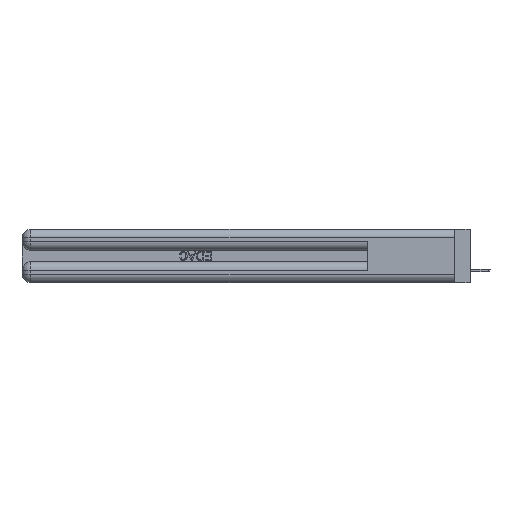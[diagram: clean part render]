
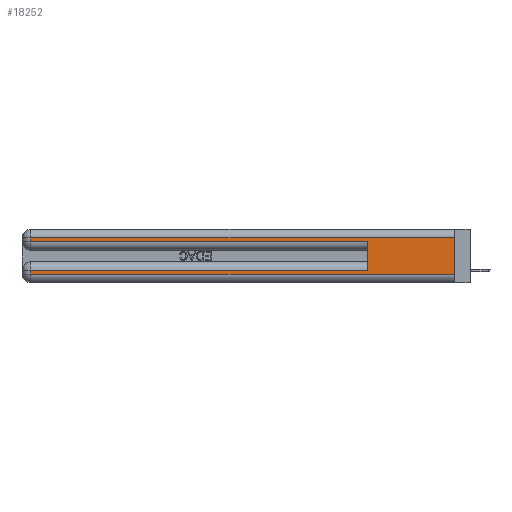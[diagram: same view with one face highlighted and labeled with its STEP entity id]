
A CAD part, left-side view. The second image highlights one B-rep face of the part: STEP entity #18252.
In plain terms, the highlighted planar face has unit normal (-1, 0, 0).
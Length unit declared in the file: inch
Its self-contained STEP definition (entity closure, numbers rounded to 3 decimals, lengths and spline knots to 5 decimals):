
#287 = LINE ( 'NONE', #26226, #33432 ) ;
#987 = DIRECTION ( 'NONE',  ( 0., 0., -1. ) ) ;
#2122 = CARTESIAN_POINT ( 'NONE',  ( 0., 0., 0.31 ) ) ;
#2546 = CARTESIAN_POINT ( 'NONE',  ( 0., 2.94, 0.085 ) ) ;
#4358 = DIRECTION ( 'NONE',  ( 0., -1., 0. ) ) ;
#5493 = DIRECTION ( 'NONE',  ( 0., 0., 1. ) ) ;
#5714 = LINE ( 'NONE', #21910, #31093 ) ;
#5759 = DIRECTION ( 'NONE',  ( 1., 0., 0. ) ) ;
#6904 = CARTESIAN_POINT ( 'NONE',  ( 0., 2.94, 0.37 ) ) ;
#7263 = ORIENTED_EDGE ( 'NONE', *, *, #36534, .T. ) ;
#8748 = ORIENTED_EDGE ( 'NONE', *, *, #12127, .F. ) ;
#9732 = EDGE_CURVE ( 'NONE', #21792, #30166, #13409, .T. ) ;
#9757 = VECTOR ( 'NONE', #29922, 39.37008 ) ;
#9833 = ORIENTED_EDGE ( 'NONE', *, *, #31726, .F. ) ;
#10038 = VERTEX_POINT ( 'NONE', #2122 ) ;
#10102 = LINE ( 'NONE', #6904, #31248 ) ;
#10202 = DIRECTION ( 'NONE',  ( 0., 1., 0. ) ) ;
#10518 = ORIENTED_EDGE ( 'NONE', *, *, #30777, .T. ) ;
#10985 = CARTESIAN_POINT ( 'NONE',  ( 0., 0., 0.37 ) ) ;
#11195 = DIRECTION ( 'NONE',  ( 0., 0., -1. ) ) ;
#11714 = VERTEX_POINT ( 'NONE', #38288 ) ;
#12050 = VECTOR ( 'NONE', #32093, 39.37008 ) ;
#12127 = EDGE_CURVE ( 'NONE', #21792, #15154, #5714, .T. ) ;
#12878 = ORIENTED_EDGE ( 'NONE', *, *, #9732, .T. ) ;
#13328 = VERTEX_POINT ( 'NONE', #26686 ) ;
#13409 = LINE ( 'NONE', #39317, #22171 ) ;
#13779 = LINE ( 'NONE', #10985, #36702 ) ;
#13881 = CARTESIAN_POINT ( 'NONE',  ( 0., 0.6, 0.085 ) ) ;
#15154 = VERTEX_POINT ( 'NONE', #39203 ) ;
#15973 = CARTESIAN_POINT ( 'NONE',  ( 0., 0., 0.37 ) ) ;
#16172 = CARTESIAN_POINT ( 'NONE',  ( 0., 2.94, 0.31 ) ) ;
#16539 = ORIENTED_EDGE ( 'NONE', *, *, #23867, .T. ) ;
#18048 = EDGE_LOOP ( 'NONE', ( #9833, #7263, #10518, #16539, #8748, #12878, #34590, #31144 ) ) ;
#18252 = ADVANCED_FACE ( 'NONE', ( #41254 ), #18977, .F. ) ;
#18642 = VERTEX_POINT ( 'NONE', #31468 ) ;
#18977 = PLANE ( 'NONE',  #26817 ) ;
#19143 = CARTESIAN_POINT ( 'NONE',  ( 0., 0., 0.285 ) ) ;
#21792 = VERTEX_POINT ( 'NONE', #13881 ) ;
#21910 = CARTESIAN_POINT ( 'NONE',  ( 0., 0.6, 0.145 ) ) ;
#22171 = VECTOR ( 'NONE', #10202, 39.37008 ) ;
#23328 = CARTESIAN_POINT ( 'NONE',  ( 0., 0., 0.31 ) ) ;
#23867 = EDGE_CURVE ( 'NONE', #13328, #15154, #35286, .T. ) ;
#24806 = VECTOR ( 'NONE', #4358, 39.37008 ) ;
#26226 = CARTESIAN_POINT ( 'NONE',  ( 0., 2.94, 0.37 ) ) ;
#26686 = CARTESIAN_POINT ( 'NONE',  ( 0., 2.94, 0.285 ) ) ;
#26753 = LINE ( 'NONE', #23328, #9757 ) ;
#26817 = AXIS2_PLACEMENT_3D ( 'NONE', #15973, #5759, #31719 ) ;
#29922 = DIRECTION ( 'NONE',  ( 0., 1., 0. ) ) ;
#30166 = VERTEX_POINT ( 'NONE', #2546 ) ;
#30777 = EDGE_CURVE ( 'NONE', #40948, #13328, #10102, .T. ) ;
#31093 = VECTOR ( 'NONE', #5493, 39.37008 ) ;
#31144 = ORIENTED_EDGE ( 'NONE', *, *, #38515, .T. ) ;
#31248 = VECTOR ( 'NONE', #987, 39.37008 ) ;
#31468 = CARTESIAN_POINT ( 'NONE',  ( 0., 0., 0.06 ) ) ;
#31719 = DIRECTION ( 'NONE',  ( 0., 0., -1. ) ) ;
#31726 = EDGE_CURVE ( 'NONE', #10038, #18642, #13779, .T. ) ;
#32093 = DIRECTION ( 'NONE',  ( 0., -1., 0. ) ) ;
#33432 = VECTOR ( 'NONE', #39134, 39.37008 ) ;
#33488 = CARTESIAN_POINT ( 'NONE',  ( 0., 0., 0.06 ) ) ;
#34590 = ORIENTED_EDGE ( 'NONE', *, *, #35662, .T. ) ;
#35286 = LINE ( 'NONE', #19143, #12050 ) ;
#35662 = EDGE_CURVE ( 'NONE', #30166, #11714, #287, .T. ) ;
#36534 = EDGE_CURVE ( 'NONE', #10038, #40948, #26753, .T. ) ;
#36702 = VECTOR ( 'NONE', #11195, 39.37008 ) ;
#38288 = CARTESIAN_POINT ( 'NONE',  ( 0., 2.94, 0.06 ) ) ;
#38515 = EDGE_CURVE ( 'NONE', #11714, #18642, #40684, .T. ) ;
#39134 = DIRECTION ( 'NONE',  ( 0., 0., -1. ) ) ;
#39203 = CARTESIAN_POINT ( 'NONE',  ( 0., 0.6, 0.285 ) ) ;
#39317 = CARTESIAN_POINT ( 'NONE',  ( 0., 0., 0.085 ) ) ;
#40684 = LINE ( 'NONE', #33488, #24806 ) ;
#40948 = VERTEX_POINT ( 'NONE', #16172 ) ;
#41254 = FACE_OUTER_BOUND ( 'NONE', #18048, .T. ) ;
